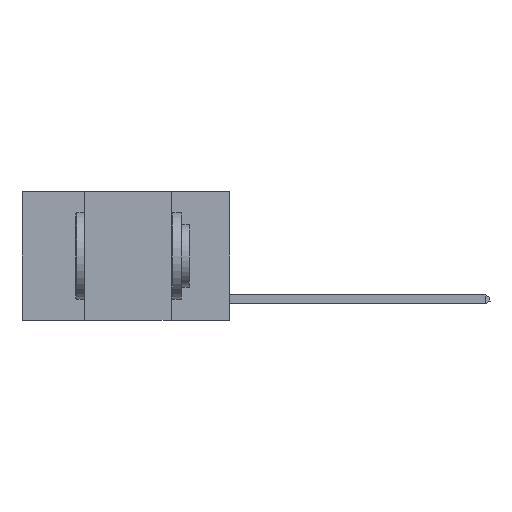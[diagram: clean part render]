
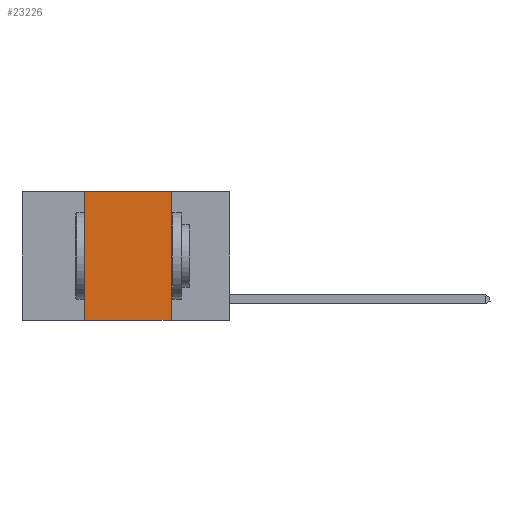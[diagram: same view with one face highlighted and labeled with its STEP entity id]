
A CAD part, left-side view. The second image highlights one B-rep face of the part: STEP entity #23226.
In plain terms, the highlighted planar face has unit normal (-1, 0, 0).
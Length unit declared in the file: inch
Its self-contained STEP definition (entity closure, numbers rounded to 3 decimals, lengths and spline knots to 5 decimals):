
#1496 = LINE ( 'NONE', #20477, #18722 ) ;
#3489 = EDGE_CURVE ( 'NONE', #3919, #15415, #4991, .T. ) ;
#3919 = VERTEX_POINT ( 'NONE', #26344 ) ;
#4991 = LINE ( 'NONE', #22091, #22858 ) ;
#5002 = EDGE_CURVE ( 'NONE', #15415, #21080, #23851, .T. ) ;
#6106 = CARTESIAN_POINT ( 'NONE',  ( 0., 0.42, -0.37 ) ) ;
#6531 = CARTESIAN_POINT ( 'NONE',  ( 0., 0.17, 0. ) ) ;
#8664 = ORIENTED_EDGE ( 'NONE', *, *, #5002, .F. ) ;
#8696 = ORIENTED_EDGE ( 'NONE', *, *, #3489, .F. ) ;
#8887 = DIRECTION ( 'NONE',  ( 0., 0., -1. ) ) ;
#8930 = DIRECTION ( 'NONE',  ( 0., 0., 1. ) ) ;
#9389 = ORIENTED_EDGE ( 'NONE', *, *, #23920, .F. ) ;
#10101 = EDGE_LOOP ( 'NONE', ( #8664, #8696, #9389, #17188 ) ) ;
#10516 = DIRECTION ( 'NONE',  ( 0., -1., 0. ) ) ;
#11533 = VECTOR ( 'NONE', #8887, 39.37008 ) ;
#13491 = AXIS2_PLACEMENT_3D ( 'NONE', #13678, #29847, #15979 ) ;
#13678 = CARTESIAN_POINT ( 'NONE',  ( 0., 0.6, 0. ) ) ;
#13991 = VECTOR ( 'NONE', #28613, 39.37008 ) ;
#15415 = VERTEX_POINT ( 'NONE', #16371 ) ;
#15590 = EDGE_CURVE ( 'NONE', #24446, #21080, #20836, .T. ) ;
#15979 = DIRECTION ( 'NONE',  ( 0., 0., -1. ) ) ;
#16371 = CARTESIAN_POINT ( 'NONE',  ( 0., 0.17, 0. ) ) ;
#17188 = ORIENTED_EDGE ( 'NONE', *, *, #15590, .T. ) ;
#18722 = VECTOR ( 'NONE', #8930, 39.37008 ) ;
#20161 = CARTESIAN_POINT ( 'NONE',  ( 0., 0.17, -0.37 ) ) ;
#20477 = CARTESIAN_POINT ( 'NONE',  ( 0., 0.42, 0. ) ) ;
#20836 = LINE ( 'NONE', #21626, #13991 ) ;
#21080 = VERTEX_POINT ( 'NONE', #20161 ) ;
#21626 = CARTESIAN_POINT ( 'NONE',  ( 0., 0.6, -0.37 ) ) ;
#22091 = CARTESIAN_POINT ( 'NONE',  ( 0., 0.6, 0. ) ) ;
#22858 = VECTOR ( 'NONE', #10516, 39.37008 ) ;
#23226 = ADVANCED_FACE ( 'NONE', ( #26048 ), #27529, .F. ) ;
#23851 = LINE ( 'NONE', #6531, #11533 ) ;
#23920 = EDGE_CURVE ( 'NONE', #24446, #3919, #1496, .T. ) ;
#24446 = VERTEX_POINT ( 'NONE', #6106 ) ;
#26048 = FACE_OUTER_BOUND ( 'NONE', #10101, .T. ) ;
#26344 = CARTESIAN_POINT ( 'NONE',  ( 0., 0.42, 0. ) ) ;
#27529 = PLANE ( 'NONE',  #13491 ) ;
#28613 = DIRECTION ( 'NONE',  ( 0., -1., 0. ) ) ;
#29847 = DIRECTION ( 'NONE',  ( 1., 0., 0. ) ) ;
